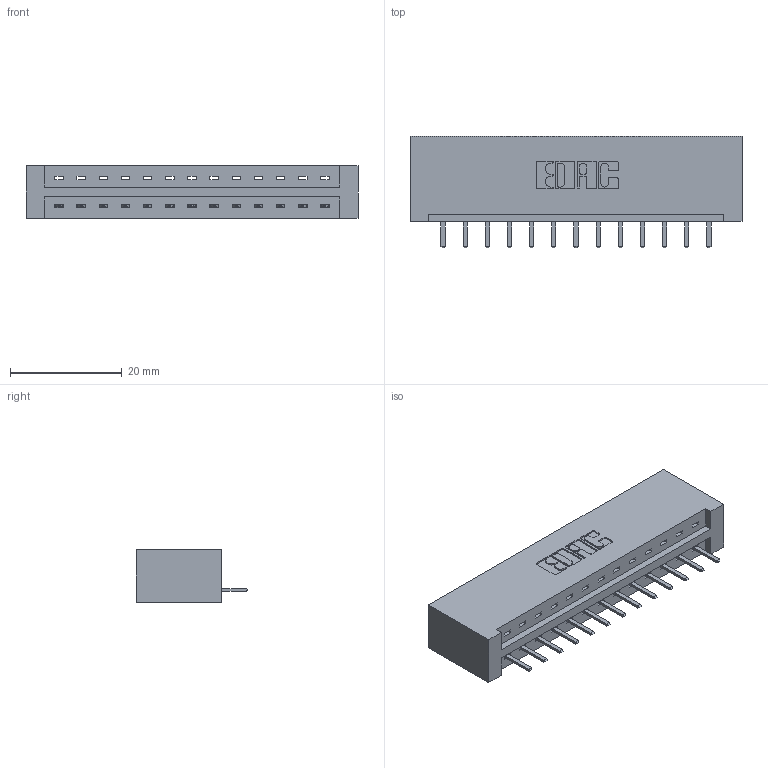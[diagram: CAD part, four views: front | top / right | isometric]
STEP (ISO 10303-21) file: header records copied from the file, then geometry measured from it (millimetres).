
FILE_DESCRIPTION (( 'STEP AP203' ), '1' );
FILE_NAME ('387-013-520-101.STEP', '2019-10-02T13:48:43', ( '' ), ( '' ), 'SwSTEP 2.0', 'SolidWorks 2016', '' );
FILE_SCHEMA (( 'CONFIG_CONTROL_DESIGN' ));
Length unit declared in the file: inch
Products named in the file (3): 387-013-520-101; 337 Part_No Mounting Lugs; 345-292-001_345-293-120
Assembly tree (14 placements, depth 2):
  387-013-520-101
    337 Part_No Mounting Lugs
    345-292-001_345-293-120  x13
Bounding box: 59.39 x 20.02 x 9.4 mm (x, y, z)
Volume: 6510.5 mm3; surface area: 6413.5 mm2
Topology: 14 solids, 14 shells, 964 faces, 2835 edges, 1854 vertices
Faces by surface type: plane 690, cylinder 274
Entity records: 13251 total; most frequent: CARTESIAN_POINT 2325, ORIENTED_EDGE 2262, DIRECTION 1997, EDGE_CURVE 1131, VECTOR 1007, LINE 1007, VERTEX_POINT 750, AXIS2_PLACEMENT_3D 495
